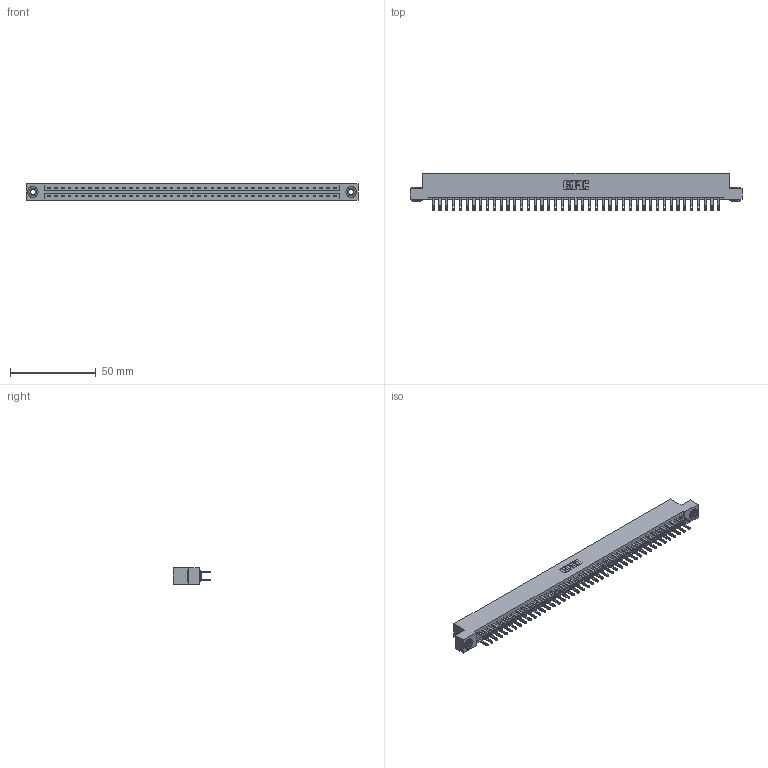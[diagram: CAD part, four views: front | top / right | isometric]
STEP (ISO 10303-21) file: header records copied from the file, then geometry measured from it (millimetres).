
FILE_DESCRIPTION (( 'STEP AP203' ), '1' );
FILE_NAME ('337-086-500-203.STEP', '2018-08-13T00:08:32', ( '' ), ( '' ), 'SwSTEP 2.0', 'SolidWorks 2016', '' );
FILE_SCHEMA (( 'CONFIG_CONTROL_DESIGN' ));
Length unit declared in the file: inch
Products named in the file (4): 337 Part_Flush Mounting Lugs - 0.156 Dia-TH; 345-292-001_345-293-100; 345-250-002_345-250-002-102; 337-086-500-203
Assembly tree (89 placements, depth 2):
  337-086-500-203
    337 Part_Flush Mounting Lugs - 0.156 Dia-TH
    345-292-001_345-293-100  x86
    345-250-002_345-250-002-102  x2
Bounding box: 193.4 x 21.85 x 9.4 mm (x, y, z)
Volume: 20677.1 mm3; surface area: 24563.8 mm2
Topology: 89 solids, 89 shells, 4452 faces, 13545 edges, 9026 vertices
Faces by surface type: plane 2832, cylinder 1612, cone 8
Entity records: 33790 total; most frequent: CARTESIAN_POINT 5665, ORIENTED_EDGE 5594, DIRECTION 4851, EDGE_CURVE 2797, VECTOR 2641, LINE 2641, VERTEX_POINT 1862, AXIS2_PLACEMENT_3D 1105
